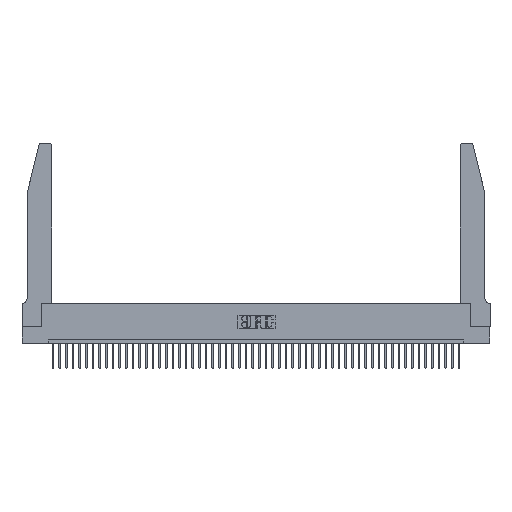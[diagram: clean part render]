
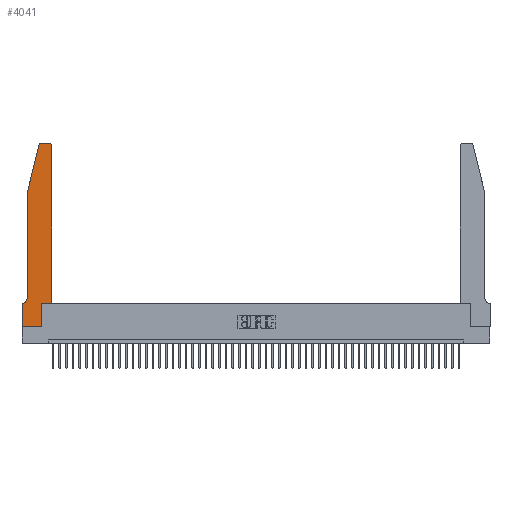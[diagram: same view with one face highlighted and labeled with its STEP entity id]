
A CAD part, top view. The second image highlights one B-rep face of the part: STEP entity #4041.
In plain terms, the highlighted planar face has unit normal (0, 0, 1).
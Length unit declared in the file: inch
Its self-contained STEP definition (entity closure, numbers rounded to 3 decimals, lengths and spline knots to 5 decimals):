
#159 = VERTEX_POINT ( 'NONE', #3270 ) ;
#961 = ORIENTED_EDGE ( 'NONE', *, *, #42724, .T. ) ;
#1134 = CIRCLE ( 'NONE', #34951, 0.03 ) ;
#1216 = CARTESIAN_POINT ( 'NONE',  ( 0., 0., 0.37 ) ) ;
#1823 = VECTOR ( 'NONE', #8057, 39.37008 ) ;
#2590 = CARTESIAN_POINT ( 'NONE',  ( 0.4205, 2.72, 0.37 ) ) ;
#3108 = ORIENTED_EDGE ( 'NONE', *, *, #24556, .T. ) ;
#3270 = CARTESIAN_POINT ( 'NONE',  ( 0.0755, 0.42, 0.37 ) ) ;
#3291 = VERTEX_POINT ( 'NONE', #39748 ) ;
#3292 = CARTESIAN_POINT ( 'NONE',  ( 0.284, 2.75, 0.37 ) ) ;
#3603 = VECTOR ( 'NONE', #19308, 39.37008 ) ;
#4041 = ADVANCED_FACE ( 'NONE', ( #8808 ), #33474, .T. ) ;
#4590 = CARTESIAN_POINT ( 'NONE',  ( 0.4505, 0.35, 0.37 ) ) ;
#4766 = ORIENTED_EDGE ( 'NONE', *, *, #9623, .T. ) ;
#5342 = LINE ( 'NONE', #1216, #3603 ) ;
#6734 = DIRECTION ( 'NONE',  ( 0., 0., -1. ) ) ;
#7402 = DIRECTION ( 'NONE',  ( 0., 1., 0. ) ) ;
#8057 = DIRECTION ( 'NONE',  ( -1., 0., 0. ) ) ;
#8409 = CARTESIAN_POINT ( 'NONE',  ( 0.2865, 0., 0.37 ) ) ;
#8485 = DIRECTION ( 'NONE',  ( -1., 0., 0. ) ) ;
#8717 = VERTEX_POINT ( 'NONE', #32523 ) ;
#8799 = DIRECTION ( 'NONE',  ( 1., 0., 0. ) ) ;
#8808 = FACE_OUTER_BOUND ( 'NONE', #29084, .T. ) ;
#8958 = CARTESIAN_POINT ( 'NONE',  ( 0., 0., 0.37 ) ) ;
#9623 = EDGE_CURVE ( 'NONE', #8717, #41581, #46629, .T. ) ;
#10227 = DIRECTION ( 'NONE',  ( 0., -1., 0. ) ) ;
#10851 = LINE ( 'NONE', #33126, #48578 ) ;
#10963 = VERTEX_POINT ( 'NONE', #38939 ) ;
#10992 = CARTESIAN_POINT ( 'NONE',  ( 0.4505, 0.35, 0.37 ) ) ;
#12672 = VECTOR ( 'NONE', #39626, 39.37008 ) ;
#13203 = ORIENTED_EDGE ( 'NONE', *, *, #14392, .T. ) ;
#14080 = CARTESIAN_POINT ( 'NONE',  ( 0., 0., 0.37 ) ) ;
#14392 = EDGE_CURVE ( 'NONE', #26477, #40643, #36880, .T. ) ;
#14732 = VECTOR ( 'NONE', #37811, 39.37008 ) ;
#14850 = CARTESIAN_POINT ( 'NONE',  ( 0., 0.35, 0.37 ) ) ;
#16395 = LINE ( 'NONE', #48426, #34094 ) ;
#18623 = CARTESIAN_POINT ( 'NONE',  ( 0.0755, 0.35, 0.37 ) ) ;
#18742 = DIRECTION ( 'NONE',  ( 1., 0., 0. ) ) ;
#19308 = DIRECTION ( 'NONE',  ( 0., -1., 0. ) ) ;
#21345 = DIRECTION ( 'NONE',  ( 0., 1., 0. ) ) ;
#21498 = DIRECTION ( 'NONE',  ( 1., 0., 0. ) ) ;
#22099 = VERTEX_POINT ( 'NONE', #8409 ) ;
#23454 = CARTESIAN_POINT ( 'NONE',  ( 0.2605, 2.75, 0.37 ) ) ;
#24556 = EDGE_CURVE ( 'NONE', #33481, #159, #10851, .T. ) ;
#24700 = LINE ( 'NONE', #26520, #14732 ) ;
#24785 = CIRCLE ( 'NONE', #32314, 0.03 ) ;
#24895 = DIRECTION ( 'NONE',  ( 0., 0., 1. ) ) ;
#25375 = CARTESIAN_POINT ( 'NONE',  ( 0.284, 2.72, 0.37 ) ) ;
#26430 = CARTESIAN_POINT ( 'NONE',  ( 0.4505, 2.72, 0.37 ) ) ;
#26477 = VERTEX_POINT ( 'NONE', #10992 ) ;
#26520 = CARTESIAN_POINT ( 'NONE',  ( 0.0755, 2., 0.37 ) ) ;
#26662 = ORIENTED_EDGE ( 'NONE', *, *, #40985, .T. ) ;
#26818 = VERTEX_POINT ( 'NONE', #14080 ) ;
#27668 = ORIENTED_EDGE ( 'NONE', *, *, #29174, .T. ) ;
#28050 = CARTESIAN_POINT ( 'NONE',  ( 0.4205, 2.75, 0.37 ) ) ;
#28169 = EDGE_CURVE ( 'NONE', #22099, #10963, #16395, .T. ) ;
#28172 = VERTEX_POINT ( 'NONE', #3292 ) ;
#29084 = EDGE_LOOP ( 'NONE', ( #961, #46562, #31397, #3108, #43365, #4766, #43157, #27668, #36311, #43697, #13203, #26662 ) ) ;
#29174 = EDGE_CURVE ( 'NONE', #26818, #22099, #31212, .T. ) ;
#29402 = CARTESIAN_POINT ( 'NONE',  ( 0.0055, 0.42, 0.37 ) ) ;
#29616 = DIRECTION ( 'NONE',  ( 0., 0., 1. ) ) ;
#31212 = LINE ( 'NONE', #8958, #38906 ) ;
#31397 = ORIENTED_EDGE ( 'NONE', *, *, #41138, .T. ) ;
#32314 = AXIS2_PLACEMENT_3D ( 'NONE', #25375, #24895, #47824 ) ;
#32523 = CARTESIAN_POINT ( 'NONE',  ( 0.0055, 0.35, 0.37 ) ) ;
#32702 = EDGE_CURVE ( 'NONE', #10963, #26477, #42775, .T. ) ;
#33080 = DIRECTION ( 'NONE',  ( -1., 0., 0. ) ) ;
#33126 = CARTESIAN_POINT ( 'NONE',  ( 0.0755, 2., 0.37 ) ) ;
#33474 = PLANE ( 'NONE',  #41676 ) ;
#33481 = VERTEX_POINT ( 'NONE', #39509 ) ;
#33713 = AXIS2_PLACEMENT_3D ( 'NONE', #29402, #6734, #33080 ) ;
#34094 = VECTOR ( 'NONE', #7402, 39.37008 ) ;
#34795 = EDGE_CURVE ( 'NONE', #28172, #3291, #24785, .T. ) ;
#34951 = AXIS2_PLACEMENT_3D ( 'NONE', #2590, #37020, #21498 ) ;
#35017 = VECTOR ( 'NONE', #21345, 39.37008 ) ;
#36311 = ORIENTED_EDGE ( 'NONE', *, *, #28169, .T. ) ;
#36880 = LINE ( 'NONE', #43982, #35017 ) ;
#37020 = DIRECTION ( 'NONE',  ( 0., 0., 1. ) ) ;
#37811 = DIRECTION ( 'NONE',  ( -0.239, -0.971, 0. ) ) ;
#38835 = VECTOR ( 'NONE', #8485, 39.37008 ) ;
#38906 = VECTOR ( 'NONE', #8799, 39.37008 ) ;
#38939 = CARTESIAN_POINT ( 'NONE',  ( 0.2865, 0.35, 0.37 ) ) ;
#39350 = EDGE_CURVE ( 'NONE', #159, #8717, #40253, .T. ) ;
#39509 = CARTESIAN_POINT ( 'NONE',  ( 0.0755, 2., 0.37 ) ) ;
#39626 = DIRECTION ( 'NONE',  ( 1., 0., 0. ) ) ;
#39748 = CARTESIAN_POINT ( 'NONE',  ( 0.25487, 2.72718, 0.37 ) ) ;
#40253 = CIRCLE ( 'NONE', #33713, 0.07 ) ;
#40643 = VERTEX_POINT ( 'NONE', #26430 ) ;
#40985 = EDGE_CURVE ( 'NONE', #40643, #45223, #1134, .T. ) ;
#41138 = EDGE_CURVE ( 'NONE', #3291, #33481, #24700, .T. ) ;
#41232 = LINE ( 'NONE', #23454, #38835 ) ;
#41581 = VERTEX_POINT ( 'NONE', #47662 ) ;
#41676 = AXIS2_PLACEMENT_3D ( 'NONE', #14850, #29616, #18742 ) ;
#42724 = EDGE_CURVE ( 'NONE', #45223, #28172, #41232, .T. ) ;
#42775 = LINE ( 'NONE', #4590, #12672 ) ;
#43157 = ORIENTED_EDGE ( 'NONE', *, *, #48680, .T. ) ;
#43365 = ORIENTED_EDGE ( 'NONE', *, *, #39350, .T. ) ;
#43697 = ORIENTED_EDGE ( 'NONE', *, *, #32702, .T. ) ;
#43982 = CARTESIAN_POINT ( 'NONE',  ( 0.4505, 0.35, 0.37 ) ) ;
#45223 = VERTEX_POINT ( 'NONE', #28050 ) ;
#46562 = ORIENTED_EDGE ( 'NONE', *, *, #34795, .T. ) ;
#46629 = LINE ( 'NONE', #18623, #1823 ) ;
#47662 = CARTESIAN_POINT ( 'NONE',  ( 0., 0.35, 0.37 ) ) ;
#47824 = DIRECTION ( 'NONE',  ( 1., 0., 0. ) ) ;
#48426 = CARTESIAN_POINT ( 'NONE',  ( 0.2865, 0.35, 0.37 ) ) ;
#48578 = VECTOR ( 'NONE', #10227, 39.37008 ) ;
#48680 = EDGE_CURVE ( 'NONE', #41581, #26818, #5342, .T. ) ;
